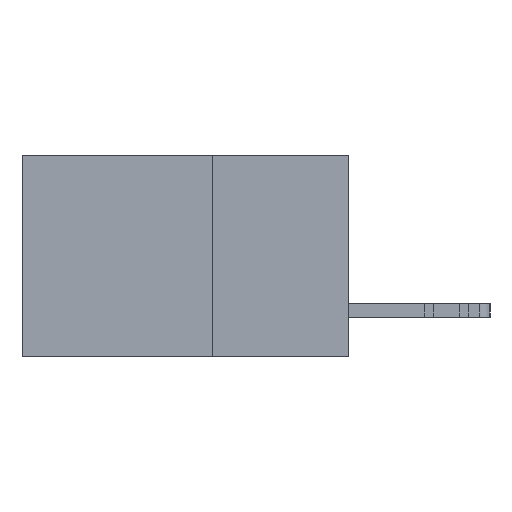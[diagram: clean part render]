
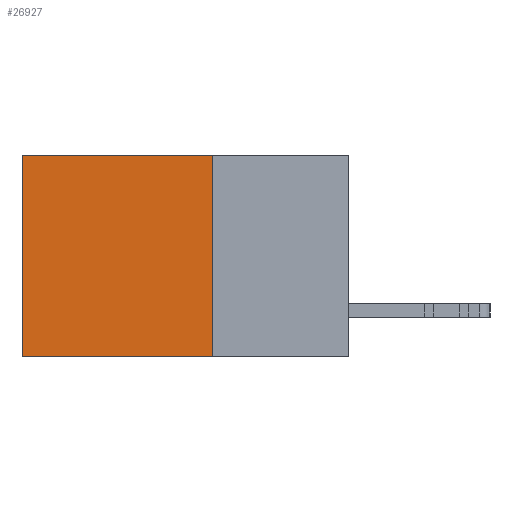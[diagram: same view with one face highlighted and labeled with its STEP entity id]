
A CAD part, left-side view. The second image highlights one B-rep face of the part: STEP entity #26927.
In plain terms, the highlighted planar face has unit normal (-1, 0, 0).
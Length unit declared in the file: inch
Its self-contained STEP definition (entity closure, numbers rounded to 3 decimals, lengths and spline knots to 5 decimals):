
#1077 = DIRECTION ( 'NONE',  ( 0., 1., 0. ) ) ;
#1839 = LINE ( 'NONE', #25194, #27400 ) ;
#5547 = EDGE_LOOP ( 'NONE', ( #25001, #10990, #19766, #20914 ) ) ;
#6666 = PLANE ( 'NONE',  #28281 ) ;
#7378 = FACE_OUTER_BOUND ( 'NONE', #5547, .T. ) ;
#8987 = CARTESIAN_POINT ( 'NONE',  ( 0.298, 0.25, 0. ) ) ;
#9094 = DIRECTION ( 'NONE',  ( 0., 0., -1. ) ) ;
#9154 = VECTOR ( 'NONE', #1077, 39.37008 ) ;
#9300 = VECTOR ( 'NONE', #22220, 39.37008 ) ;
#9321 = VERTEX_POINT ( 'NONE', #19839 ) ;
#10515 = CARTESIAN_POINT ( 'NONE',  ( 0.298, 0.25, 0. ) ) ;
#10713 = EDGE_CURVE ( 'NONE', #22254, #16147, #1839, .T. ) ;
#10832 = DIRECTION ( 'NONE',  ( 0., 0., -1. ) ) ;
#10990 = ORIENTED_EDGE ( 'NONE', *, *, #30306, .F. ) ;
#13070 = LINE ( 'NONE', #28782, #26287 ) ;
#14421 = DIRECTION ( 'NONE',  ( 0., 0., -1. ) ) ;
#15530 = LINE ( 'NONE', #27350, #9154 ) ;
#16050 = VERTEX_POINT ( 'NONE', #21914 ) ;
#16147 = VERTEX_POINT ( 'NONE', #22218 ) ;
#18117 = EDGE_CURVE ( 'NONE', #9321, #16050, #13070, .T. ) ;
#19508 = EDGE_CURVE ( 'NONE', #22254, #9321, #24332, .T. ) ;
#19766 = ORIENTED_EDGE ( 'NONE', *, *, #10713, .F. ) ;
#19813 = CARTESIAN_POINT ( 'NONE',  ( 0.298, 0.25, 0. ) ) ;
#19839 = CARTESIAN_POINT ( 'NONE',  ( 0.298, 0.6, 0. ) ) ;
#20914 = ORIENTED_EDGE ( 'NONE', *, *, #19508, .T. ) ;
#21914 = CARTESIAN_POINT ( 'NONE',  ( 0.298, 0.6, -0.37 ) ) ;
#22218 = CARTESIAN_POINT ( 'NONE',  ( 0.298, 0.25, -0.37 ) ) ;
#22220 = DIRECTION ( 'NONE',  ( 0., 1., 0. ) ) ;
#22254 = VERTEX_POINT ( 'NONE', #10515 ) ;
#23465 = DIRECTION ( 'NONE',  ( 1., 0., 0. ) ) ;
#24332 = LINE ( 'NONE', #19813, #9300 ) ;
#25001 = ORIENTED_EDGE ( 'NONE', *, *, #18117, .T. ) ;
#25194 = CARTESIAN_POINT ( 'NONE',  ( 0.298, 0.25, 0. ) ) ;
#26287 = VECTOR ( 'NONE', #14421, 39.37008 ) ;
#26927 = ADVANCED_FACE ( 'NONE', ( #7378 ), #6666, .F. ) ;
#27350 = CARTESIAN_POINT ( 'NONE',  ( 0.298, 0.25, -0.37 ) ) ;
#27400 = VECTOR ( 'NONE', #10832, 39.37008 ) ;
#28281 = AXIS2_PLACEMENT_3D ( 'NONE', #8987, #23465, #9094 ) ;
#28782 = CARTESIAN_POINT ( 'NONE',  ( 0.298, 0.6, 0. ) ) ;
#30306 = EDGE_CURVE ( 'NONE', #16147, #16050, #15530, .T. ) ;
